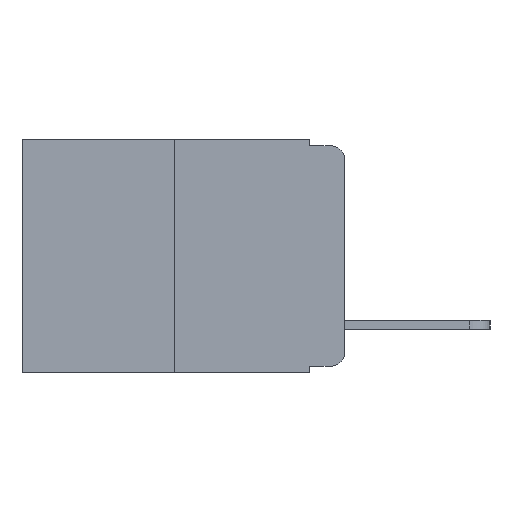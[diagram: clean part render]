
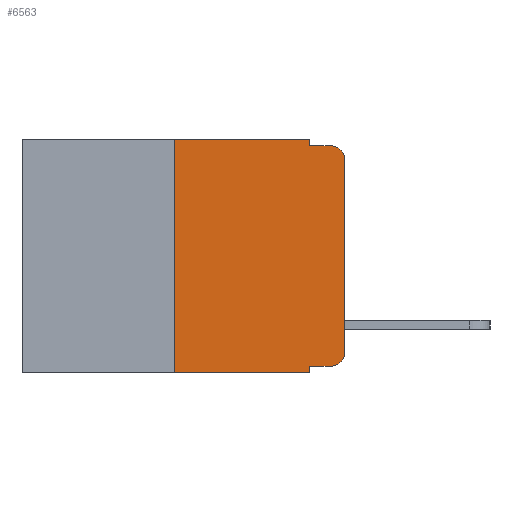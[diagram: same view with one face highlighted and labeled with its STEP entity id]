
A CAD part, left-side view. The second image highlights one B-rep face of the part: STEP entity #6563.
In plain terms, the highlighted planar face has unit normal (-1, 0, 0).
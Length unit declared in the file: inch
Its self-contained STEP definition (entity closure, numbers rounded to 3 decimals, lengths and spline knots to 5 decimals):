
#292 = LINE ( 'NONE', #10983, #10616 ) ;
#700 = ORIENTED_EDGE ( 'NONE', *, *, #10074, .T. ) ;
#740 = DIRECTION ( 'NONE',  ( 0., 0., 1. ) ) ;
#793 = DIRECTION ( 'NONE',  ( 0., 0., -1. ) ) ;
#798 = CARTESIAN_POINT ( 'NONE',  ( 0., 0.051, 0. ) ) ;
#832 = ORIENTED_EDGE ( 'NONE', *, *, #11277, .F. ) ;
#1122 = CARTESIAN_POINT ( 'NONE',  ( 0., 0.25, 0. ) ) ;
#1400 = DIRECTION ( 'NONE',  ( 0., -1., 0. ) ) ;
#1439 = CARTESIAN_POINT ( 'NONE',  ( 0., 0.051, -0.01 ) ) ;
#1476 = DIRECTION ( 'NONE',  ( 0., 0., -1. ) ) ;
#1509 = DIRECTION ( 'NONE',  ( -1., 0., 0. ) ) ;
#1559 = CARTESIAN_POINT ( 'NONE',  ( 0., 0.02, -0.03 ) ) ;
#1786 = DIRECTION ( 'NONE',  ( 0., 0., 1. ) ) ;
#1880 = CARTESIAN_POINT ( 'NONE',  ( 0., 0., 0. ) ) ;
#1897 = ORIENTED_EDGE ( 'NONE', *, *, #11068, .F. ) ;
#2009 = VERTEX_POINT ( 'NONE', #3312 ) ;
#2052 = CARTESIAN_POINT ( 'NONE',  ( 0., 0.02, -0.01 ) ) ;
#2236 = DIRECTION ( 'NONE',  ( 0., -1., 0. ) ) ;
#2323 = CARTESIAN_POINT ( 'NONE',  ( 0., 0.473, 0. ) ) ;
#2857 = ORIENTED_EDGE ( 'NONE', *, *, #11294, .T. ) ;
#3312 = CARTESIAN_POINT ( 'NONE',  ( 0., 0.25, -0.343 ) ) ;
#3356 = CARTESIAN_POINT ( 'NONE',  ( 0., 0.051, -0.01 ) ) ;
#3393 = CARTESIAN_POINT ( 'NONE',  ( 0., 0.02, -0.333 ) ) ;
#3445 = CARTESIAN_POINT ( 'NONE',  ( 0., 0., -0.313 ) ) ;
#3738 = LINE ( 'NONE', #1880, #9732 ) ;
#3751 = VERTEX_POINT ( 'NONE', #10856 ) ;
#3935 = CIRCLE ( 'NONE', #5046, 0.02 ) ;
#4030 = ORIENTED_EDGE ( 'NONE', *, *, #11299, .T. ) ;
#4518 = AXIS2_PLACEMENT_3D ( 'NONE', #1559, #1509, #1476 ) ;
#4696 = VERTEX_POINT ( 'NONE', #3356 ) ;
#4761 = CARTESIAN_POINT ( 'NONE',  ( 0., 0.051, 0. ) ) ;
#5046 = AXIS2_PLACEMENT_3D ( 'NONE', #9669, #9955, #9640 ) ;
#5149 = LINE ( 'NONE', #8100, #10627 ) ;
#5358 = VERTEX_POINT ( 'NONE', #4761 ) ;
#5403 = VERTEX_POINT ( 'NONE', #3445 ) ;
#5512 = LINE ( 'NONE', #12451, #10255 ) ;
#5895 = VECTOR ( 'NONE', #740, 39.37008 ) ;
#6014 = VERTEX_POINT ( 'NONE', #3393 ) ;
#6262 = VECTOR ( 'NONE', #1400, 39.37008 ) ;
#6563 = ADVANCED_FACE ( 'NONE', ( #10476 ), #14569, .F. ) ;
#6736 = CARTESIAN_POINT ( 'NONE',  ( 0., 0.051, -0.333 ) ) ;
#6758 = VERTEX_POINT ( 'NONE', #13060 ) ;
#7631 = EDGE_CURVE ( 'NONE', #3751, #5358, #9108, .T. ) ;
#7959 = DIRECTION ( 'NONE',  ( 0., -1., 0. ) ) ;
#8100 = CARTESIAN_POINT ( 'NONE',  ( 0., 0.473, -0.343 ) ) ;
#8150 = ORIENTED_EDGE ( 'NONE', *, *, #11020, .T. ) ;
#8403 = VERTEX_POINT ( 'NONE', #6736 ) ;
#8991 = VERTEX_POINT ( 'NONE', #14362 ) ;
#9079 = VECTOR ( 'NONE', #793, 39.37008 ) ;
#9108 = LINE ( 'NONE', #2323, #14309 ) ;
#9640 = DIRECTION ( 'NONE',  ( 0., 0., -1. ) ) ;
#9669 = CARTESIAN_POINT ( 'NONE',  ( 0., 0.02, -0.313 ) ) ;
#9711 = ORIENTED_EDGE ( 'NONE', *, *, #11023, .T. ) ;
#9732 = VECTOR ( 'NONE', #1786, 39.37008 ) ;
#9955 = DIRECTION ( 'NONE',  ( -1., 0., 0. ) ) ;
#10074 = EDGE_CURVE ( 'NONE', #2009, #8991, #5149, .T. ) ;
#10075 = ORIENTED_EDGE ( 'NONE', *, *, #11040, .F. ) ;
#10255 = VECTOR ( 'NONE', #12035, 39.37008 ) ;
#10476 = FACE_OUTER_BOUND ( 'NONE', #11736, .T. ) ;
#10616 = VECTOR ( 'NONE', #10991, 39.37008 ) ;
#10627 = VECTOR ( 'NONE', #7959, 39.37008 ) ;
#10856 = CARTESIAN_POINT ( 'NONE',  ( 0., 0.25, 0. ) ) ;
#10950 = ORIENTED_EDGE ( 'NONE', *, *, #11064, .F. ) ;
#10983 = CARTESIAN_POINT ( 'NONE',  ( 0., 0.051, -0.333 ) ) ;
#10991 = DIRECTION ( 'NONE',  ( 0., -1., 0. ) ) ;
#11020 = EDGE_CURVE ( 'NONE', #5403, #6758, #3738, .T. ) ;
#11023 = EDGE_CURVE ( 'NONE', #6758, #12757, #12214, .T. ) ;
#11040 = EDGE_CURVE ( 'NONE', #4696, #12757, #14607, .T. ) ;
#11064 = EDGE_CURVE ( 'NONE', #5358, #4696, #11608, .T. ) ;
#11068 = EDGE_CURVE ( 'NONE', #2009, #3751, #14284, .T. ) ;
#11277 = EDGE_CURVE ( 'NONE', #8403, #8991, #5512, .T. ) ;
#11294 = EDGE_CURVE ( 'NONE', #8403, #6014, #292, .T. ) ;
#11299 = EDGE_CURVE ( 'NONE', #6014, #5403, #3935, .T. ) ;
#11319 = ORIENTED_EDGE ( 'NONE', *, *, #7631, .F. ) ;
#11608 = LINE ( 'NONE', #798, #9079 ) ;
#11736 = EDGE_LOOP ( 'NONE', ( #8150, #9711, #10075, #10950, #11319, #1897, #700, #832, #2857, #4030 ) ) ;
#12035 = DIRECTION ( 'NONE',  ( 0., 0., -1. ) ) ;
#12214 = CIRCLE ( 'NONE', #4518, 0.02 ) ;
#12451 = CARTESIAN_POINT ( 'NONE',  ( 0., 0.051, 0. ) ) ;
#12757 = VERTEX_POINT ( 'NONE', #2052 ) ;
#13060 = CARTESIAN_POINT ( 'NONE',  ( 0., 0., -0.03 ) ) ;
#14284 = LINE ( 'NONE', #1122, #5895 ) ;
#14309 = VECTOR ( 'NONE', #2236, 39.37008 ) ;
#14362 = CARTESIAN_POINT ( 'NONE',  ( 0., 0.051, -0.343 ) ) ;
#14460 = DIRECTION ( 'NONE',  ( 0., 0., -1. ) ) ;
#14501 = DIRECTION ( 'NONE',  ( 1., 0., 0. ) ) ;
#14536 = CARTESIAN_POINT ( 'NONE',  ( 0., 0.473, 0. ) ) ;
#14555 = AXIS2_PLACEMENT_3D ( 'NONE', #14536, #14501, #14460 ) ;
#14569 = PLANE ( 'NONE',  #14555 ) ;
#14607 = LINE ( 'NONE', #1439, #6262 ) ;
